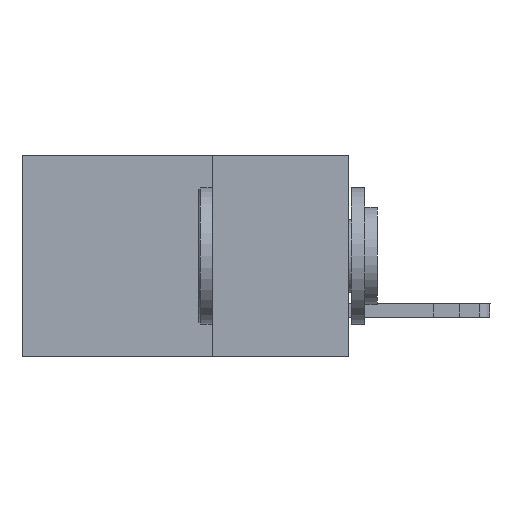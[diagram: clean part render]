
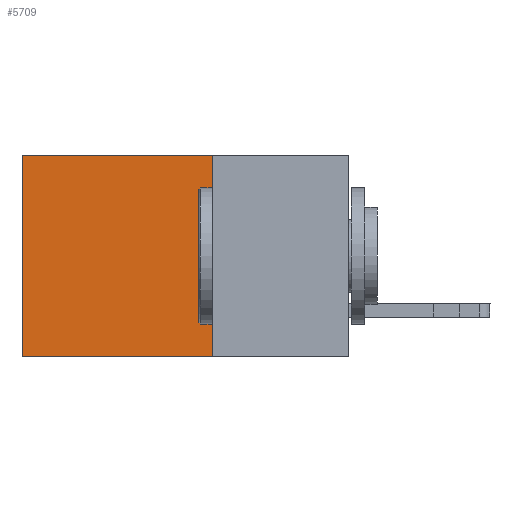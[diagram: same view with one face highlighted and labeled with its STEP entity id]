
A CAD part, left-side view. The second image highlights one B-rep face of the part: STEP entity #5709.
In plain terms, the highlighted planar face has unit normal (-1, 0, 0).
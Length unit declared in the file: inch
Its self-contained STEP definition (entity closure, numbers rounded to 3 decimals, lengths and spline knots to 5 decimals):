
#739 = VERTEX_POINT ( 'NONE', #14034 ) ;
#1627 = ORIENTED_EDGE ( 'NONE', *, *, #7987, .F. ) ;
#2305 = ORIENTED_EDGE ( 'NONE', *, *, #7759, .T. ) ;
#2358 = AXIS2_PLACEMENT_3D ( 'NONE', #12524, #5751, #8047 ) ;
#2449 = DIRECTION ( 'NONE',  ( 0., 1., 0. ) ) ;
#2588 = EDGE_CURVE ( 'NONE', #5745, #739, #5563, .T. ) ;
#3574 = PLANE ( 'NONE',  #2358 ) ;
#3680 = EDGE_CURVE ( 'NONE', #13393, #12105, #11896, .T. ) ;
#3783 = VECTOR ( 'NONE', #9394, 39.37008 ) ;
#4837 = CARTESIAN_POINT ( 'NONE',  ( 0.298, 0.6, 0. ) ) ;
#4855 = ORIENTED_EDGE ( 'NONE', *, *, #3680, .F. ) ;
#5522 = VECTOR ( 'NONE', #10687, 39.37008 ) ;
#5563 = LINE ( 'NONE', #4837, #3783 ) ;
#5709 = ADVANCED_FACE ( 'NONE', ( #7896 ), #3574, .F. ) ;
#5745 = VERTEX_POINT ( 'NONE', #8144 ) ;
#5751 = DIRECTION ( 'NONE',  ( 1., 0., 0. ) ) ;
#6308 = CARTESIAN_POINT ( 'NONE',  ( 0.298, 0.25, 0. ) ) ;
#7480 = DIRECTION ( 'NONE',  ( 0., 1., 0. ) ) ;
#7490 = VECTOR ( 'NONE', #7480, 39.37008 ) ;
#7759 = EDGE_CURVE ( 'NONE', #13393, #5745, #12241, .T. ) ;
#7896 = FACE_OUTER_BOUND ( 'NONE', #11078, .T. ) ;
#7987 = EDGE_CURVE ( 'NONE', #12105, #739, #13481, .T. ) ;
#8047 = DIRECTION ( 'NONE',  ( 0., 0., -1. ) ) ;
#8144 = CARTESIAN_POINT ( 'NONE',  ( 0.298, 0.6, 0. ) ) ;
#9394 = DIRECTION ( 'NONE',  ( 0., 0., -1. ) ) ;
#10687 = DIRECTION ( 'NONE',  ( 0., 0., -1. ) ) ;
#11078 = EDGE_LOOP ( 'NONE', ( #12199, #1627, #4855, #2305 ) ) ;
#11896 = LINE ( 'NONE', #6308, #5522 ) ;
#12105 = VERTEX_POINT ( 'NONE', #12322 ) ;
#12199 = ORIENTED_EDGE ( 'NONE', *, *, #2588, .T. ) ;
#12241 = LINE ( 'NONE', #13047, #7490 ) ;
#12322 = CARTESIAN_POINT ( 'NONE',  ( 0.298, 0.25, -0.37 ) ) ;
#12524 = CARTESIAN_POINT ( 'NONE',  ( 0.298, 0.25, 0. ) ) ;
#12709 = CARTESIAN_POINT ( 'NONE',  ( 0.298, 0.25, -0.37 ) ) ;
#13047 = CARTESIAN_POINT ( 'NONE',  ( 0.298, 0.25, 0. ) ) ;
#13393 = VERTEX_POINT ( 'NONE', #14343 ) ;
#13481 = LINE ( 'NONE', #12709, #14204 ) ;
#14034 = CARTESIAN_POINT ( 'NONE',  ( 0.298, 0.6, -0.37 ) ) ;
#14204 = VECTOR ( 'NONE', #2449, 39.37008 ) ;
#14343 = CARTESIAN_POINT ( 'NONE',  ( 0.298, 0.25, 0. ) ) ;
